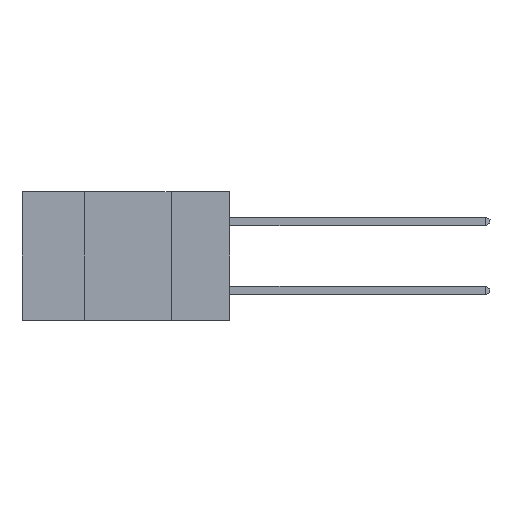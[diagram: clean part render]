
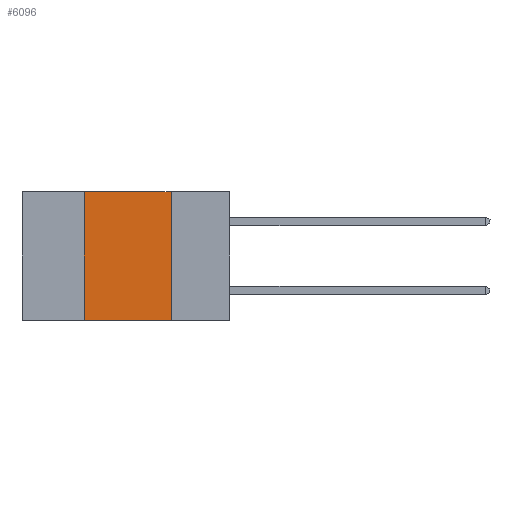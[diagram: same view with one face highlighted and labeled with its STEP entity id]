
A CAD part, left-side view. The second image highlights one B-rep face of the part: STEP entity #6096.
In plain terms, the highlighted planar face has unit normal (-1, 0, 0).
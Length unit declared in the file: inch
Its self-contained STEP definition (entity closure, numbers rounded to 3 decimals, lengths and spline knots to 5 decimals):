
#23 = VECTOR ( 'NONE', #7404, 39.37008 ) ;
#230 = EDGE_CURVE ( 'NONE', #2410, #10074, #6245, .T. ) ;
#612 = CARTESIAN_POINT ( 'NONE',  ( 0., 0.17, -0.37 ) ) ;
#710 = EDGE_CURVE ( 'NONE', #5909, #10074, #1940, .T. ) ;
#885 = DIRECTION ( 'NONE',  ( 0., 0., -1. ) ) ;
#900 = LINE ( 'NONE', #10472, #9931 ) ;
#1024 = DIRECTION ( 'NONE',  ( 0., -1., 0. ) ) ;
#1940 = LINE ( 'NONE', #2057, #3244 ) ;
#2057 = CARTESIAN_POINT ( 'NONE',  ( 0., 0.6, -0.37 ) ) ;
#2115 = CARTESIAN_POINT ( 'NONE',  ( 0., 0.42, 0. ) ) ;
#2410 = VERTEX_POINT ( 'NONE', #7262 ) ;
#2794 = ORIENTED_EDGE ( 'NONE', *, *, #10300, .F. ) ;
#2886 = DIRECTION ( 'NONE',  ( 0., 0., 1. ) ) ;
#3244 = VECTOR ( 'NONE', #1024, 39.37008 ) ;
#3606 = CARTESIAN_POINT ( 'NONE',  ( 0., 0.6, 0. ) ) ;
#3678 = ORIENTED_EDGE ( 'NONE', *, *, #710, .T. ) ;
#3718 = FACE_OUTER_BOUND ( 'NONE', #7448, .T. ) ;
#3852 = CARTESIAN_POINT ( 'NONE',  ( 0., 0.42, -0.37 ) ) ;
#4358 = DIRECTION ( 'NONE',  ( 1., 0., 0. ) ) ;
#5909 = VERTEX_POINT ( 'NONE', #3852 ) ;
#6096 = ADVANCED_FACE ( 'NONE', ( #3718 ), #10499, .F. ) ;
#6202 = VERTEX_POINT ( 'NONE', #2115 ) ;
#6245 = LINE ( 'NONE', #9505, #8657 ) ;
#6397 = LINE ( 'NONE', #3606, #23 ) ;
#7173 = DIRECTION ( 'NONE',  ( 0., 0., -1. ) ) ;
#7262 = CARTESIAN_POINT ( 'NONE',  ( 0., 0.17, 0. ) ) ;
#7404 = DIRECTION ( 'NONE',  ( 0., -1., 0. ) ) ;
#7448 = EDGE_LOOP ( 'NONE', ( #9481, #9442, #2794, #3678 ) ) ;
#8657 = VECTOR ( 'NONE', #885, 39.37008 ) ;
#8691 = CARTESIAN_POINT ( 'NONE',  ( 0., 0.6, 0. ) ) ;
#9442 = ORIENTED_EDGE ( 'NONE', *, *, #9504, .F. ) ;
#9481 = ORIENTED_EDGE ( 'NONE', *, *, #230, .F. ) ;
#9504 = EDGE_CURVE ( 'NONE', #6202, #2410, #6397, .T. ) ;
#9505 = CARTESIAN_POINT ( 'NONE',  ( 0., 0.17, -0.37 ) ) ;
#9564 = AXIS2_PLACEMENT_3D ( 'NONE', #8691, #4358, #7173 ) ;
#9931 = VECTOR ( 'NONE', #2886, 39.37008 ) ;
#10074 = VERTEX_POINT ( 'NONE', #612 ) ;
#10300 = EDGE_CURVE ( 'NONE', #5909, #6202, #900, .T. ) ;
#10472 = CARTESIAN_POINT ( 'NONE',  ( 0., 0.42, -0.37 ) ) ;
#10499 = PLANE ( 'NONE',  #9564 ) ;
